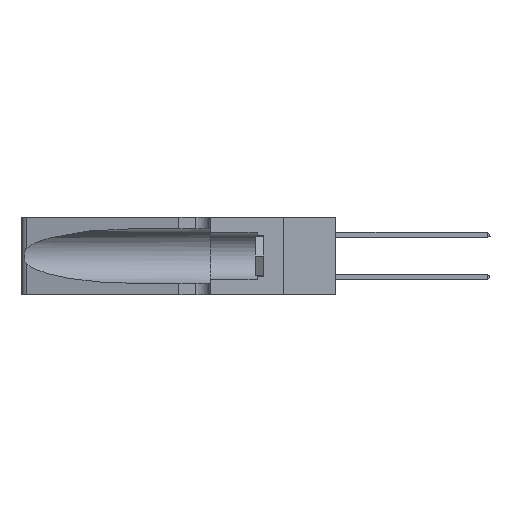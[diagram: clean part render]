
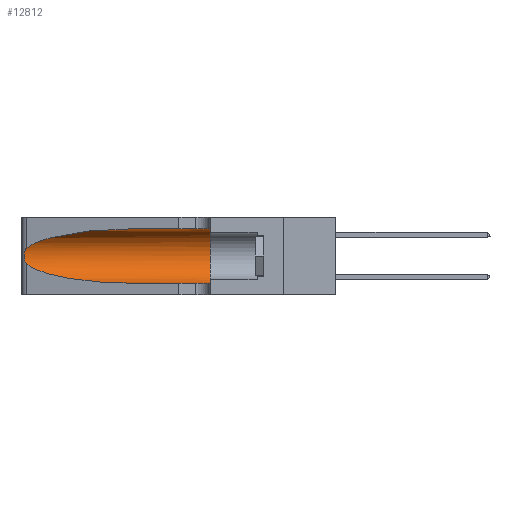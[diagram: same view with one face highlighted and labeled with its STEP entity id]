
A CAD part, left-side view. The second image highlights one B-rep face of the part: STEP entity #12812.
In plain terms, the highlighted cylindrical face has radius 3.308 mm (diameter 6.617 mm), a partial arc.
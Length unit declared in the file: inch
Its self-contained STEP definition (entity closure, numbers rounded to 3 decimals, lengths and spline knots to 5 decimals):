
#278 = VECTOR ( 'NONE', #11958, 39.37008 ) ;
#416 = VERTEX_POINT ( 'NONE', #13953 ) ;
#1101 = CARTESIAN_POINT ( 'NONE',  ( 0.26018, 1.23835, 0.19895 ) ) ;
#1455 = DIRECTION ( 'NONE',  ( 0., 0., -1. ) ) ;
#1726 = VERTEX_POINT ( 'NONE', #7984 ) ;
#2032 = ORIENTED_EDGE ( 'NONE', *, *, #4529, .T. ) ;
#2739 = CARTESIAN_POINT ( 'NONE',  ( 0.1305, 1.61858, 0.05475 ) ) ;
#2997 = EDGE_CURVE ( 'NONE', #8300, #13266, #5848, .T. ) ;
#4456 = CARTESIAN_POINT ( 'NONE',  ( 0.18966, 0.96281, 0.31525 ) ) ;
#4529 = EDGE_CURVE ( 'NONE', #6814, #416, #16925, .T. ) ;
#5050 = CARTESIAN_POINT ( 'NONE',  ( 0.25787, 1.23484, 0.2124 ) ) ;
#5197 = LINE ( 'NONE', #2739, #278 ) ;
#5848 =( BOUNDED_CURVE ( )  B_SPLINE_CURVE ( 3, ( #14621, #12926, #14702, #16357 ),
 .UNSPECIFIED., .F., .F. ) 
 B_SPLINE_CURVE_WITH_KNOTS ( ( 4, 4 ),
 ( 3.44316, 4.71239 ),
 .UNSPECIFIED. ) 
 CURVE ( )  GEOMETRIC_REPRESENTATION_ITEM ( )  RATIONAL_B_SPLINE_CURVE ( ( 1., 0.87, 0.87, 1. ) ) 
 REPRESENTATION_ITEM ( '' )  );
#6325 = CARTESIAN_POINT ( 'NONE',  ( 0.25487, 1.22718, 0.22369 ) ) ;
#6392 = AXIS2_PLACEMENT_3D ( 'NONE', #16205, #14246, #1455 ) ;
#6814 = VERTEX_POINT ( 'NONE', #7647 ) ;
#6897 = CARTESIAN_POINT ( 'NONE',  ( 0.26075, 1.23896, 0.178 ) ) ;
#7040 = CARTESIAN_POINT ( 'NONE',  ( 0.25487, 1.22718, 0.14631 ) ) ;
#7178 = DIRECTION ( 'NONE',  ( 0., 0., 1. ) ) ;
#7487 = ORIENTED_EDGE ( 'NONE', *, *, #21004, .T. ) ;
#7567 = EDGE_CURVE ( 'NONE', #6814, #1726, #8558, .T. ) ;
#7647 = CARTESIAN_POINT ( 'NONE',  ( 0.1305, 0.72297, 0.31525 ) ) ;
#7984 = CARTESIAN_POINT ( 'NONE',  ( 0.1305, 0.35, 0.31525 ) ) ;
#8300 = VERTEX_POINT ( 'NONE', #7040 ) ;
#8511 = CARTESIAN_POINT ( 'NONE',  ( 0.25555, 1.22993, 0.14849 ) ) ;
#8558 = LINE ( 'NONE', #11430, #22391 ) ;
#8582 = VERTEX_POINT ( 'NONE', #11942 ) ;
#8753 = CARTESIAN_POINT ( 'NONE',  ( 0.26017, 1.23833, 0.17102 ) ) ;
#10234 = ORIENTED_EDGE ( 'NONE', *, *, #7567, .F. ) ;
#10575 = CARTESIAN_POINT ( 'NONE',  ( 0.25487, 1.22718, 0.14631 ) ) ;
#10858 = B_SPLINE_CURVE_WITH_KNOTS ( 'NONE', 3,
 ( #12268, #12349, #16092, #5050, #12108, #1101, #15919, #6897, #8753, #23508, #13965, #21653, #8511, #10575 ),
 .UNSPECIFIED., .F., .F.,
 ( 4, 2, 2, 2, 2, 2, 4 ),
 ( 0., 0.00027, 0.00053, 0.00107, 0.0016, 0.00187, 0.00214 ),
 .UNSPECIFIED. ) ;
#11430 = CARTESIAN_POINT ( 'NONE',  ( 0.1305, 1.61858, 0.31525 ) ) ;
#11512 = EDGE_CURVE ( 'NONE', #416, #8300, #10858, .T. ) ;
#11942 = CARTESIAN_POINT ( 'NONE',  ( 0.1305, 0.35, 0.05475 ) ) ;
#11958 = DIRECTION ( 'NONE',  ( 0., -1., 0. ) ) ;
#12108 = CARTESIAN_POINT ( 'NONE',  ( 0.25854, 1.2359, 0.20912 ) ) ;
#12268 = CARTESIAN_POINT ( 'NONE',  ( 0.25487, 1.22718, 0.22369 ) ) ;
#12349 = CARTESIAN_POINT ( 'NONE',  ( 0.25555, 1.22994, 0.2215 ) ) ;
#12812 = ADVANCED_FACE ( 'NONE', ( #15452 ), #21242, .F. ) ;
#12926 = CARTESIAN_POINT ( 'NONE',  ( 0.2373, 1.15595, 0.08982 ) ) ;
#13266 = VERTEX_POINT ( 'NONE', #21339 ) ;
#13953 = CARTESIAN_POINT ( 'NONE',  ( 0.25487, 1.22718, 0.22369 ) ) ;
#13965 = CARTESIAN_POINT ( 'NONE',  ( 0.25789, 1.23486, 0.15765 ) ) ;
#14246 = DIRECTION ( 'NONE',  ( 0., -1., 0. ) ) ;
#14269 = EDGE_CURVE ( 'NONE', #1726, #8582, #19708, .T. ) ;
#14621 = CARTESIAN_POINT ( 'NONE',  ( 0.25487, 1.22718, 0.14631 ) ) ;
#14653 = CARTESIAN_POINT ( 'NONE',  ( 0.1305, 0.35, 0.185 ) ) ;
#14702 = CARTESIAN_POINT ( 'NONE',  ( 0.18966, 0.96281, 0.05475 ) ) ;
#14808 = ORIENTED_EDGE ( 'NONE', *, *, #11512, .T. ) ;
#15087 = ORIENTED_EDGE ( 'NONE', *, *, #14269, .F. ) ;
#15452 = FACE_OUTER_BOUND ( 'NONE', #22231, .T. ) ;
#15477 = CARTESIAN_POINT ( 'NONE',  ( 0.1305, 0.72297, 0.31525 ) ) ;
#15919 = CARTESIAN_POINT ( 'NONE',  ( 0.26075, 1.23896, 0.19203 ) ) ;
#16092 = CARTESIAN_POINT ( 'NONE',  ( 0.25639, 1.23184, 0.21858 ) ) ;
#16205 = CARTESIAN_POINT ( 'NONE',  ( 0.1305, 1.61858, 0.185 ) ) ;
#16303 = DIRECTION ( 'NONE',  ( 0., 1., 0. ) ) ;
#16357 = CARTESIAN_POINT ( 'NONE',  ( 0.1305, 0.72297, 0.05475 ) ) ;
#16925 =( BOUNDED_CURVE ( )  B_SPLINE_CURVE ( 3, ( #15477, #4456, #17364, #6325 ),
 .UNSPECIFIED., .F., .F. ) 
 B_SPLINE_CURVE_WITH_KNOTS ( ( 4, 4 ),
 ( 1.5708, 2.84003 ),
 .UNSPECIFIED. ) 
 CURVE ( )  GEOMETRIC_REPRESENTATION_ITEM ( )  RATIONAL_B_SPLINE_CURVE ( ( 1., 0.87, 0.87, 1. ) ) 
 REPRESENTATION_ITEM ( '' )  );
#17364 = CARTESIAN_POINT ( 'NONE',  ( 0.2373, 1.15595, 0.28018 ) ) ;
#19708 = CIRCLE ( 'NONE', #23224, 0.13025 ) ;
#20712 = DIRECTION ( 'NONE',  ( 0., -1., 0. ) ) ;
#20750 = ORIENTED_EDGE ( 'NONE', *, *, #2997, .T. ) ;
#21004 = EDGE_CURVE ( 'NONE', #13266, #8582, #5197, .T. ) ;
#21242 = CYLINDRICAL_SURFACE ( 'NONE', #6392, 0.13025 ) ;
#21339 = CARTESIAN_POINT ( 'NONE',  ( 0.1305, 0.72297, 0.05475 ) ) ;
#21653 = CARTESIAN_POINT ( 'NONE',  ( 0.25639, 1.23186, 0.15144 ) ) ;
#22231 = EDGE_LOOP ( 'NONE', ( #2032, #14808, #20750, #7487, #15087, #10234 ) ) ;
#22391 = VECTOR ( 'NONE', #20712, 39.37008 ) ;
#23224 = AXIS2_PLACEMENT_3D ( 'NONE', #14653, #16303, #7178 ) ;
#23508 = CARTESIAN_POINT ( 'NONE',  ( 0.25856, 1.23593, 0.16098 ) ) ;
